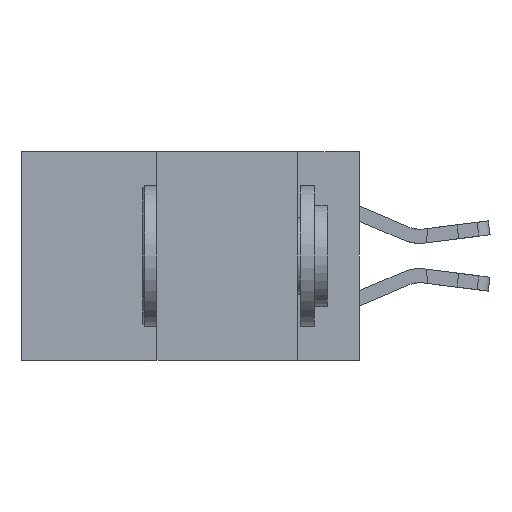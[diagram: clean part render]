
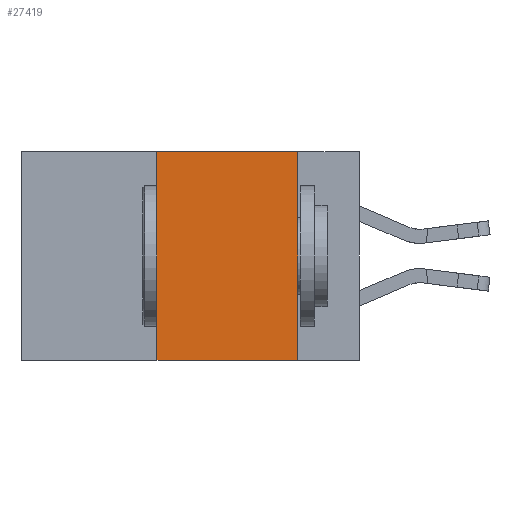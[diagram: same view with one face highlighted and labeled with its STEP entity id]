
A CAD part, left-side view. The second image highlights one B-rep face of the part: STEP entity #27419.
In plain terms, the highlighted planar face has unit normal (-1, 0, 0).
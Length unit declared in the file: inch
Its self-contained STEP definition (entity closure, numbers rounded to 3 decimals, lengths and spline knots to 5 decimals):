
#1663 = EDGE_CURVE ( 'NONE', #24670, #27696, #27480, .T. ) ;
#2862 = DIRECTION ( 'NONE',  ( 0., 0., -1. ) ) ;
#2977 = VECTOR ( 'NONE', #2862, 39.37008 ) ;
#3351 = AXIS2_PLACEMENT_3D ( 'NONE', #28032, #13409, #30495 ) ;
#3814 = LINE ( 'NONE', #13757, #10583 ) ;
#6820 = CARTESIAN_POINT ( 'NONE',  ( 0., 0.6, 0. ) ) ;
#6940 = CARTESIAN_POINT ( 'NONE',  ( 0., 0.11, -0.37 ) ) ;
#8559 = VECTOR ( 'NONE', #24076, 39.37008 ) ;
#10583 = VECTOR ( 'NONE', #30839, 39.37008 ) ;
#12295 = EDGE_CURVE ( 'NONE', #16682, #27696, #15555, .T. ) ;
#12486 = EDGE_CURVE ( 'NONE', #24670, #14188, #3814, .T. ) ;
#13210 = PLANE ( 'NONE',  #3351 ) ;
#13268 = EDGE_CURVE ( 'NONE', #14188, #16682, #26608, .T. ) ;
#13409 = DIRECTION ( 'NONE',  ( 1., 0., 0. ) ) ;
#13662 = CARTESIAN_POINT ( 'NONE',  ( 0., 0.36, -0.37 ) ) ;
#13757 = CARTESIAN_POINT ( 'NONE',  ( 0., 0.36, 0. ) ) ;
#13798 = EDGE_LOOP ( 'NONE', ( #29515, #31035, #19649, #26867 ) ) ;
#14188 = VERTEX_POINT ( 'NONE', #24687 ) ;
#15555 = LINE ( 'NONE', #20350, #2977 ) ;
#15891 = FACE_OUTER_BOUND ( 'NONE', #13798, .T. ) ;
#16682 = VERTEX_POINT ( 'NONE', #25853 ) ;
#19649 = ORIENTED_EDGE ( 'NONE', *, *, #12486, .F. ) ;
#20350 = CARTESIAN_POINT ( 'NONE',  ( 0., 0.11, 0. ) ) ;
#21571 = DIRECTION ( 'NONE',  ( 0., -1., 0. ) ) ;
#21816 = CARTESIAN_POINT ( 'NONE',  ( 0., 0.6, -0.37 ) ) ;
#24076 = DIRECTION ( 'NONE',  ( 0., -1., 0. ) ) ;
#24670 = VERTEX_POINT ( 'NONE', #13662 ) ;
#24687 = CARTESIAN_POINT ( 'NONE',  ( 0., 0.36, 0. ) ) ;
#25853 = CARTESIAN_POINT ( 'NONE',  ( 0., 0.11, 0. ) ) ;
#26608 = LINE ( 'NONE', #6820, #8559 ) ;
#26715 = VECTOR ( 'NONE', #21571, 39.37008 ) ;
#26867 = ORIENTED_EDGE ( 'NONE', *, *, #1663, .T. ) ;
#27419 = ADVANCED_FACE ( 'NONE', ( #15891 ), #13210, .F. ) ;
#27480 = LINE ( 'NONE', #21816, #26715 ) ;
#27696 = VERTEX_POINT ( 'NONE', #6940 ) ;
#28032 = CARTESIAN_POINT ( 'NONE',  ( 0., 0.6, 0. ) ) ;
#29515 = ORIENTED_EDGE ( 'NONE', *, *, #12295, .F. ) ;
#30495 = DIRECTION ( 'NONE',  ( 0., 0., -1. ) ) ;
#30839 = DIRECTION ( 'NONE',  ( 0., 0., 1. ) ) ;
#31035 = ORIENTED_EDGE ( 'NONE', *, *, #13268, .F. ) ;
